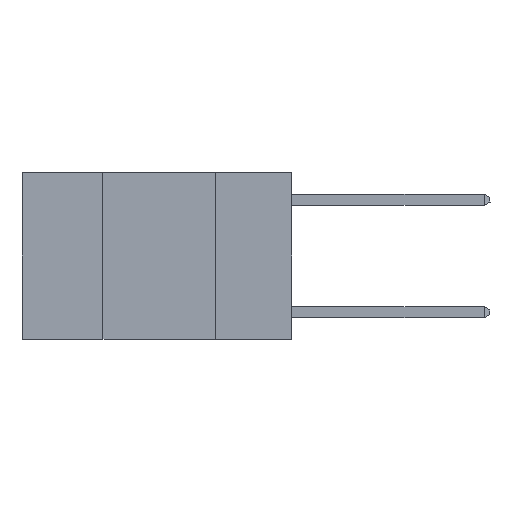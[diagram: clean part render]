
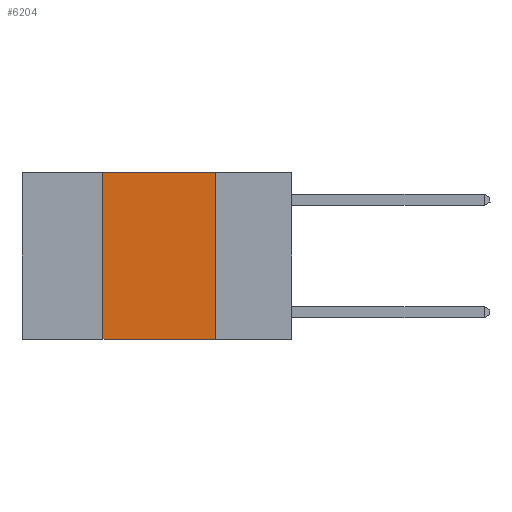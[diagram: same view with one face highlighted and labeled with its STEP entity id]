
A CAD part, left-side view. The second image highlights one B-rep face of the part: STEP entity #6204.
In plain terms, the highlighted planar face has unit normal (-1, 0, 0).
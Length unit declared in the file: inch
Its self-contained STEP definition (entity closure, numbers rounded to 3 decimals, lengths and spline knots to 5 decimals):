
#107 = VECTOR ( 'NONE', #2063, 39.37008 ) ;
#253 = AXIS2_PLACEMENT_3D ( 'NONE', #4627, #1919, #6591 ) ;
#333 = ORIENTED_EDGE ( 'NONE', *, *, #6373, .T. ) ;
#415 = VECTOR ( 'NONE', #5447, 39.37008 ) ;
#425 = VERTEX_POINT ( 'NONE', #3754 ) ;
#1103 = VERTEX_POINT ( 'NONE', #5233 ) ;
#1267 = PLANE ( 'NONE',  #253 ) ;
#1876 = LINE ( 'NONE', #4406, #5235 ) ;
#1919 = DIRECTION ( 'NONE',  ( 1., 0., 0. ) ) ;
#1922 = LINE ( 'NONE', #3395, #7065 ) ;
#2063 = DIRECTION ( 'NONE',  ( 0., 0., -1. ) ) ;
#2095 = CARTESIAN_POINT ( 'NONE',  ( 0., 0.17, 0. ) ) ;
#2649 = EDGE_LOOP ( 'NONE', ( #4343, #6604, #4799, #333 ) ) ;
#2700 = EDGE_CURVE ( 'NONE', #1103, #425, #1922, .T. ) ;
#3258 = EDGE_CURVE ( 'NONE', #425, #5658, #5648, .T. ) ;
#3395 = CARTESIAN_POINT ( 'NONE',  ( 0., 0.42, 0. ) ) ;
#3609 = CARTESIAN_POINT ( 'NONE',  ( 0., 0.6, 0. ) ) ;
#3647 = DIRECTION ( 'NONE',  ( 0., 0., 1. ) ) ;
#3754 = CARTESIAN_POINT ( 'NONE',  ( 0., 0.42, 0. ) ) ;
#4083 = FACE_OUTER_BOUND ( 'NONE', #2649, .T. ) ;
#4343 = ORIENTED_EDGE ( 'NONE', *, *, #6275, .F. ) ;
#4406 = CARTESIAN_POINT ( 'NONE',  ( 0., 0.6, -0.37 ) ) ;
#4627 = CARTESIAN_POINT ( 'NONE',  ( 0., 0.6, 0. ) ) ;
#4799 = ORIENTED_EDGE ( 'NONE', *, *, #2700, .F. ) ;
#5018 = DIRECTION ( 'NONE',  ( 0., -1., 0. ) ) ;
#5185 = CARTESIAN_POINT ( 'NONE',  ( 0., 0.17, -0.37 ) ) ;
#5233 = CARTESIAN_POINT ( 'NONE',  ( 0., 0.42, -0.37 ) ) ;
#5235 = VECTOR ( 'NONE', #5018, 39.37008 ) ;
#5447 = DIRECTION ( 'NONE',  ( 0., -1., 0. ) ) ;
#5648 = LINE ( 'NONE', #3609, #415 ) ;
#5658 = VERTEX_POINT ( 'NONE', #7008 ) ;
#6178 = VERTEX_POINT ( 'NONE', #5185 ) ;
#6204 = ADVANCED_FACE ( 'NONE', ( #4083 ), #1267, .F. ) ;
#6275 = EDGE_CURVE ( 'NONE', #5658, #6178, #6453, .T. ) ;
#6373 = EDGE_CURVE ( 'NONE', #1103, #6178, #1876, .T. ) ;
#6453 = LINE ( 'NONE', #2095, #107 ) ;
#6591 = DIRECTION ( 'NONE',  ( 0., 0., -1. ) ) ;
#6604 = ORIENTED_EDGE ( 'NONE', *, *, #3258, .F. ) ;
#7008 = CARTESIAN_POINT ( 'NONE',  ( 0., 0.17, 0. ) ) ;
#7065 = VECTOR ( 'NONE', #3647, 39.37008 ) ;
